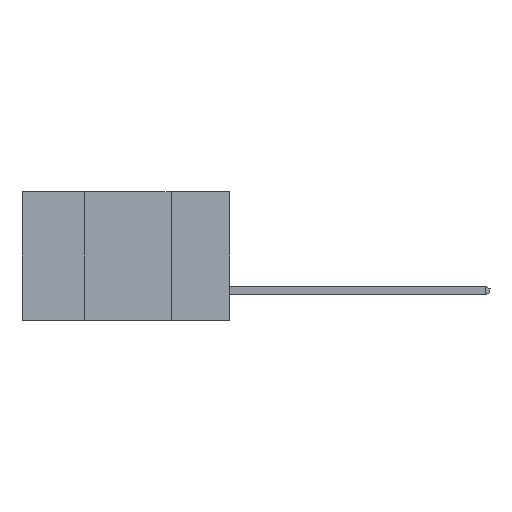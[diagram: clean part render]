
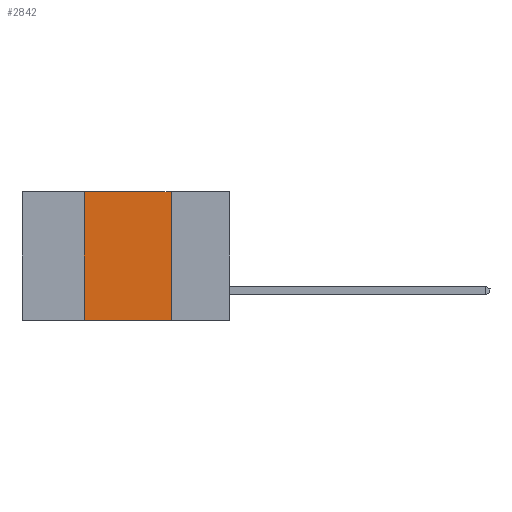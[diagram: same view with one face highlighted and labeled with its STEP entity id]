
A CAD part, left-side view. The second image highlights one B-rep face of the part: STEP entity #2842.
In plain terms, the highlighted planar face has unit normal (-1, 0, 0).
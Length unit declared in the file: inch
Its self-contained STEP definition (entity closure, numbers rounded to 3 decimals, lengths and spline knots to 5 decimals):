
#191 = EDGE_CURVE ( 'NONE', #1423, #7341, #4651, .T. ) ;
#736 = CARTESIAN_POINT ( 'NONE',  ( 0., 0.6, 0. ) ) ;
#1252 = CARTESIAN_POINT ( 'NONE',  ( 0., 0.42, 0. ) ) ;
#1423 = VERTEX_POINT ( 'NONE', #3161 ) ;
#1511 = VERTEX_POINT ( 'NONE', #1252 ) ;
#1513 = VECTOR ( 'NONE', #4697, 39.37008 ) ;
#1617 = VERTEX_POINT ( 'NONE', #8247 ) ;
#1822 = AXIS2_PLACEMENT_3D ( 'NONE', #2685, #8515, #2728 ) ;
#2152 = ORIENTED_EDGE ( 'NONE', *, *, #4748, .F. ) ;
#2180 = ORIENTED_EDGE ( 'NONE', *, *, #191, .T. ) ;
#2560 = VECTOR ( 'NONE', #6435, 39.37008 ) ;
#2648 = EDGE_CURVE ( 'NONE', #1423, #1511, #5500, .T. ) ;
#2685 = CARTESIAN_POINT ( 'NONE',  ( 0., 0.6, 0. ) ) ;
#2728 = DIRECTION ( 'NONE',  ( 0., 0., -1. ) ) ;
#2842 = ADVANCED_FACE ( 'NONE', ( #7852 ), #9379, .F. ) ;
#2988 = LINE ( 'NONE', #5276, #4031 ) ;
#3129 = DIRECTION ( 'NONE',  ( 0., 0., -1. ) ) ;
#3161 = CARTESIAN_POINT ( 'NONE',  ( 0., 0.42, -0.37 ) ) ;
#3165 = DIRECTION ( 'NONE',  ( 0., 0., 1. ) ) ;
#3364 = VECTOR ( 'NONE', #3165, 39.37008 ) ;
#4031 = VECTOR ( 'NONE', #3129, 39.37008 ) ;
#4090 = CARTESIAN_POINT ( 'NONE',  ( 0., 0.17, -0.37 ) ) ;
#4163 = EDGE_LOOP ( 'NONE', ( #2152, #9418, #7250, #2180 ) ) ;
#4646 = EDGE_CURVE ( 'NONE', #1511, #1617, #9440, .T. ) ;
#4651 = LINE ( 'NONE', #4750, #1513 ) ;
#4697 = DIRECTION ( 'NONE',  ( 0., -1., 0. ) ) ;
#4748 = EDGE_CURVE ( 'NONE', #1617, #7341, #2988, .T. ) ;
#4750 = CARTESIAN_POINT ( 'NONE',  ( 0., 0.6, -0.37 ) ) ;
#5276 = CARTESIAN_POINT ( 'NONE',  ( 0., 0.17, -0.37 ) ) ;
#5500 = LINE ( 'NONE', #8367, #3364 ) ;
#6435 = DIRECTION ( 'NONE',  ( 0., -1., 0. ) ) ;
#7250 = ORIENTED_EDGE ( 'NONE', *, *, #2648, .F. ) ;
#7341 = VERTEX_POINT ( 'NONE', #4090 ) ;
#7852 = FACE_OUTER_BOUND ( 'NONE', #4163, .T. ) ;
#8247 = CARTESIAN_POINT ( 'NONE',  ( 0., 0.17, 0. ) ) ;
#8367 = CARTESIAN_POINT ( 'NONE',  ( 0., 0.42, -0.37 ) ) ;
#8515 = DIRECTION ( 'NONE',  ( 1., 0., 0. ) ) ;
#9379 = PLANE ( 'NONE',  #1822 ) ;
#9418 = ORIENTED_EDGE ( 'NONE', *, *, #4646, .F. ) ;
#9440 = LINE ( 'NONE', #736, #2560 ) ;
